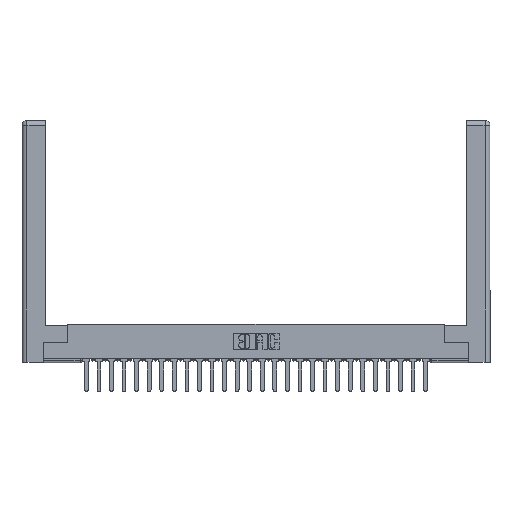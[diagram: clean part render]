
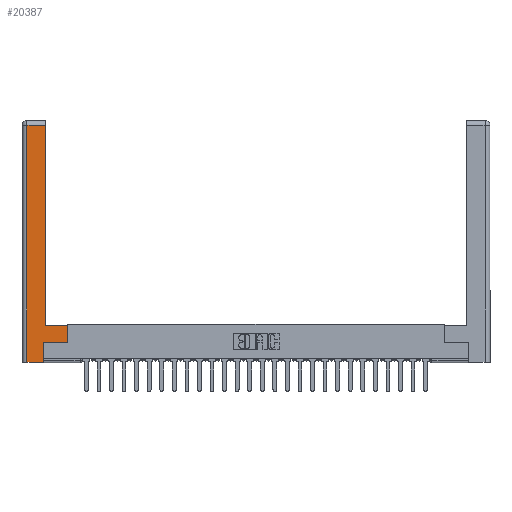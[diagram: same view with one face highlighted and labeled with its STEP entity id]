
A CAD part, top view. The second image highlights one B-rep face of the part: STEP entity #20387.
In plain terms, the highlighted planar face has unit normal (0, 0, 1).
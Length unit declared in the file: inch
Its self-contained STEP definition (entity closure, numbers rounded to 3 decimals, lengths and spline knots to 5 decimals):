
#416 = PLANE ( 'NONE',  #6959 ) ;
#1441 = DIRECTION ( 'NONE',  ( 1., 0., 0. ) ) ;
#2408 = ORIENTED_EDGE ( 'NONE', *, *, #27812, .T. ) ;
#3015 = CARTESIAN_POINT ( 'NONE',  ( 0.265, 0.245, 0. ) ) ;
#3414 = VECTOR ( 'NONE', #22530, 39.37008 ) ;
#3416 = EDGE_CURVE ( 'NONE', #6145, #4247, #17293, .T. ) ;
#3800 = CARTESIAN_POINT ( 'NONE',  ( 0.0615, 2.94, 0. ) ) ;
#3917 = EDGE_CURVE ( 'NONE', #10826, #4474, #6848, .T. ) ;
#4247 = VERTEX_POINT ( 'NONE', #28463 ) ;
#4474 = VERTEX_POINT ( 'NONE', #27525 ) ;
#5012 = FACE_OUTER_BOUND ( 'NONE', #9285, .T. ) ;
#6145 = VERTEX_POINT ( 'NONE', #16377 ) ;
#6185 = CARTESIAN_POINT ( 'NONE',  ( 0.265, 0., 0. ) ) ;
#6289 = VERTEX_POINT ( 'NONE', #3015 ) ;
#6294 = CARTESIAN_POINT ( 'NONE',  ( 0.565, 0.245, 0. ) ) ;
#6371 = LINE ( 'NONE', #6294, #11461 ) ;
#6848 = LINE ( 'NONE', #11159, #12909 ) ;
#6959 = AXIS2_PLACEMENT_3D ( 'NONE', #7389, #7677, #9901 ) ;
#7092 = VECTOR ( 'NONE', #17292, 39.37008 ) ;
#7166 = VERTEX_POINT ( 'NONE', #11965 ) ;
#7389 = CARTESIAN_POINT ( 'NONE',  ( 0., 0., 0. ) ) ;
#7677 = DIRECTION ( 'NONE',  ( 0., 0., -1. ) ) ;
#8252 = CARTESIAN_POINT ( 'NONE',  ( 0.265, 0.245, 0. ) ) ;
#8892 = DIRECTION ( 'NONE',  ( 1., 0., 0. ) ) ;
#9059 = ORIENTED_EDGE ( 'NONE', *, *, #11911, .T. ) ;
#9285 = EDGE_LOOP ( 'NONE', ( #10033, #20529, #21210, #20924, #12914, #9059, #2408, #11775 ) ) ;
#9636 = EDGE_CURVE ( 'NONE', #4247, #27915, #25986, .T. ) ;
#9901 = DIRECTION ( 'NONE',  ( -1., 0., 0. ) ) ;
#10033 = ORIENTED_EDGE ( 'NONE', *, *, #28432, .T. ) ;
#10386 = EDGE_CURVE ( 'NONE', #27915, #16681, #26487, .T. ) ;
#10826 = VERTEX_POINT ( 'NONE', #20810 ) ;
#11159 = CARTESIAN_POINT ( 'NONE',  ( 0.295, 0.45, 0. ) ) ;
#11461 = VECTOR ( 'NONE', #8892, 39.37008 ) ;
#11592 = CARTESIAN_POINT ( 'NONE',  ( 0.0615, 0., 0. ) ) ;
#11775 = ORIENTED_EDGE ( 'NONE', *, *, #3917, .T. ) ;
#11911 = EDGE_CURVE ( 'NONE', #6289, #7166, #6371, .T. ) ;
#11965 = CARTESIAN_POINT ( 'NONE',  ( 0.565, 0.245, 0. ) ) ;
#12564 = DIRECTION ( 'NONE',  ( -1., 0., 0. ) ) ;
#12909 = VECTOR ( 'NONE', #20466, 39.37008 ) ;
#12914 = ORIENTED_EDGE ( 'NONE', *, *, #25978, .T. ) ;
#14266 = VECTOR ( 'NONE', #15044, 39.37008 ) ;
#14748 = LINE ( 'NONE', #26435, #14266 ) ;
#15044 = DIRECTION ( 'NONE',  ( 0., 1., 0. ) ) ;
#15346 = CARTESIAN_POINT ( 'NONE',  ( 0.0615, 0., 0. ) ) ;
#16377 = CARTESIAN_POINT ( 'NONE',  ( 0.295, 2.94, 0. ) ) ;
#16681 = VERTEX_POINT ( 'NONE', #20533 ) ;
#17146 = LINE ( 'NONE', #8252, #7092 ) ;
#17292 = DIRECTION ( 'NONE',  ( 0., 1., 0. ) ) ;
#17293 = LINE ( 'NONE', #3800, #23720 ) ;
#20387 = ADVANCED_FACE ( 'NONE', ( #5012 ), #416, .F. ) ;
#20466 = DIRECTION ( 'NONE',  ( -1., 0., 0. ) ) ;
#20529 = ORIENTED_EDGE ( 'NONE', *, *, #3416, .T. ) ;
#20533 = CARTESIAN_POINT ( 'NONE',  ( 0.265, 0., 0. ) ) ;
#20810 = CARTESIAN_POINT ( 'NONE',  ( 0.565, 0.45, 0. ) ) ;
#20840 = VECTOR ( 'NONE', #22011, 39.37008 ) ;
#20924 = ORIENTED_EDGE ( 'NONE', *, *, #10386, .T. ) ;
#21210 = ORIENTED_EDGE ( 'NONE', *, *, #9636, .T. ) ;
#21326 = VECTOR ( 'NONE', #1441, 39.37008 ) ;
#22011 = DIRECTION ( 'NONE',  ( 0., -1., 0. ) ) ;
#22530 = DIRECTION ( 'NONE',  ( 0., 1., 0. ) ) ;
#23720 = VECTOR ( 'NONE', #12564, 39.37008 ) ;
#24891 = CARTESIAN_POINT ( 'NONE',  ( 0.295, 3., 0. ) ) ;
#25978 = EDGE_CURVE ( 'NONE', #16681, #6289, #17146, .T. ) ;
#25986 = LINE ( 'NONE', #15346, #20840 ) ;
#26435 = CARTESIAN_POINT ( 'NONE',  ( 0.565, 0.45, 0. ) ) ;
#26487 = LINE ( 'NONE', #6185, #21326 ) ;
#27525 = CARTESIAN_POINT ( 'NONE',  ( 0.295, 0.45, 0. ) ) ;
#27812 = EDGE_CURVE ( 'NONE', #7166, #10826, #14748, .T. ) ;
#27915 = VERTEX_POINT ( 'NONE', #11592 ) ;
#28432 = EDGE_CURVE ( 'NONE', #4474, #6145, #28902, .T. ) ;
#28463 = CARTESIAN_POINT ( 'NONE',  ( 0.0615, 2.94, 0. ) ) ;
#28902 = LINE ( 'NONE', #24891, #3414 ) ;
